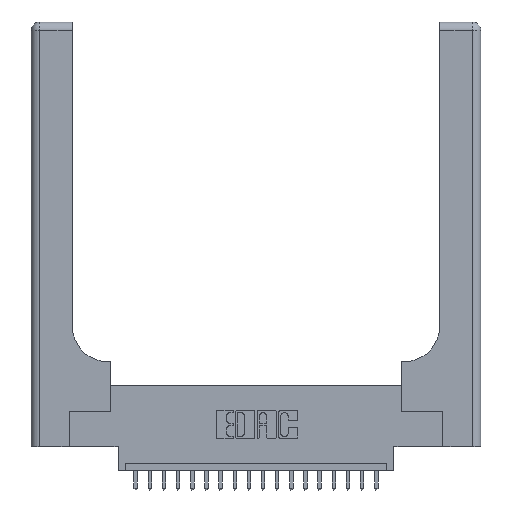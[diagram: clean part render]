
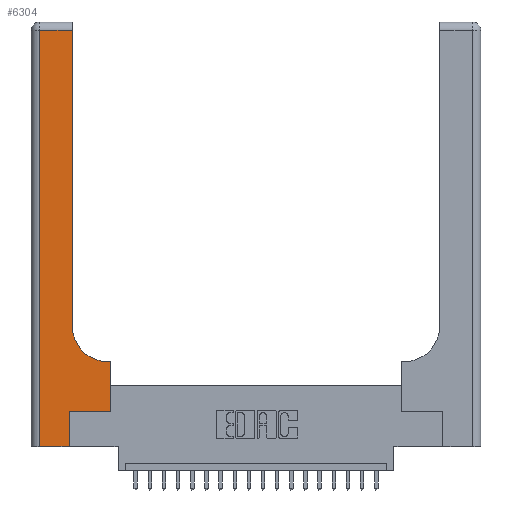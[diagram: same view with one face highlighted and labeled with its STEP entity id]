
A CAD part, top view. The second image highlights one B-rep face of the part: STEP entity #6304.
In plain terms, the highlighted planar face has unit normal (0, 0, 1).
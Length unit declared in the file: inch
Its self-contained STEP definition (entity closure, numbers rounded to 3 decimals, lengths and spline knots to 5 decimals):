
#1231 = CARTESIAN_POINT ( 'NONE',  ( 0.2915, 0.6, 0.37 ) ) ;
#1843 = CARTESIAN_POINT ( 'NONE',  ( 0.5585, 0.25, 0.37 ) ) ;
#1884 = DIRECTION ( 'NONE',  ( 1., 0., 0. ) ) ;
#3087 = VERTEX_POINT ( 'NONE', #7261 ) ;
#3095 = CARTESIAN_POINT ( 'NONE',  ( 0., 0., 0.37 ) ) ;
#3444 = EDGE_CURVE ( 'NONE', #20006, #18761, #9945, .T. ) ;
#3661 = ORIENTED_EDGE ( 'NONE', *, *, #21456, .T. ) ;
#4259 = EDGE_CURVE ( 'NONE', #7028, #18705, #18725, .T. ) ;
#4614 = VECTOR ( 'NONE', #9133, 39.37008 ) ;
#4795 = EDGE_CURVE ( 'NONE', #3087, #5387, #10986, .T. ) ;
#5135 = LINE ( 'NONE', #1843, #13689 ) ;
#5152 = EDGE_LOOP ( 'NONE', ( #8022, #11754, #18284, #7652, #18877, #15872, #3661, #17086, #14059 ) ) ;
#5387 = VERTEX_POINT ( 'NONE', #13367 ) ;
#5657 = VECTOR ( 'NONE', #9217, 39.37008 ) ;
#5728 = VERTEX_POINT ( 'NONE', #8145 ) ;
#5735 = CARTESIAN_POINT ( 'NONE',  ( 0.2915, 3., 0.37 ) ) ;
#5755 = EDGE_CURVE ( 'NONE', #18761, #3087, #11507, .T. ) ;
#5797 = DIRECTION ( 'NONE',  ( -1., 0., 0. ) ) ;
#5877 = VECTOR ( 'NONE', #9684, 39.37008 ) ;
#6205 = VECTOR ( 'NONE', #18537, 39.37008 ) ;
#6304 = ADVANCED_FACE ( 'NONE', ( #13922 ), #12515, .F. ) ;
#7028 = VERTEX_POINT ( 'NONE', #10907 ) ;
#7101 = DIRECTION ( 'NONE',  ( 0., 1., 0. ) ) ;
#7230 = DIRECTION ( 'NONE',  ( 1., 0., 0. ) ) ;
#7261 = CARTESIAN_POINT ( 'NONE',  ( 0.269, 0., 0.37 ) ) ;
#7466 = CARTESIAN_POINT ( 'NONE',  ( 0.5415, 0.85, 0.37 ) ) ;
#7652 = ORIENTED_EDGE ( 'NONE', *, *, #5755, .T. ) ;
#8022 = ORIENTED_EDGE ( 'NONE', *, *, #4259, .T. ) ;
#8145 = CARTESIAN_POINT ( 'NONE',  ( 0.5415, 0.6, 0.37 ) ) ;
#8517 = VERTEX_POINT ( 'NONE', #21505 ) ;
#9133 = DIRECTION ( 'NONE',  ( 0., 1., 0. ) ) ;
#9148 = DIRECTION ( 'NONE',  ( 0., 0., -1. ) ) ;
#9217 = DIRECTION ( 'NONE',  ( 0., 1., 0. ) ) ;
#9305 = VERTEX_POINT ( 'NONE', #10525 ) ;
#9640 = CARTESIAN_POINT ( 'NONE',  ( 0.06, 0., 0.37 ) ) ;
#9684 = DIRECTION ( 'NONE',  ( -1., 0., 0. ) ) ;
#9945 = LINE ( 'NONE', #13618, #6205 ) ;
#10200 = CIRCLE ( 'NONE', #17585, 0.25 ) ;
#10267 = DIRECTION ( 'NONE',  ( -1., 0., 0. ) ) ;
#10525 = CARTESIAN_POINT ( 'NONE',  ( 0.5585, 0.6, 0.37 ) ) ;
#10907 = CARTESIAN_POINT ( 'NONE',  ( 0.2915, 0.85, 0.37 ) ) ;
#10986 = LINE ( 'NONE', #17590, #4614 ) ;
#11022 = DIRECTION ( 'NONE',  ( 0., 0., -1. ) ) ;
#11041 = CARTESIAN_POINT ( 'NONE',  ( 0.06, 2.94, 0.37 ) ) ;
#11507 = LINE ( 'NONE', #3095, #16042 ) ;
#11711 = EDGE_CURVE ( 'NONE', #9305, #5728, #20611, .T. ) ;
#11749 = CARTESIAN_POINT ( 'NONE',  ( 0., 3., 0.37 ) ) ;
#11754 = ORIENTED_EDGE ( 'NONE', *, *, #12599, .T. ) ;
#12015 = EDGE_CURVE ( 'NONE', #5387, #8517, #20897, .T. ) ;
#12515 = PLANE ( 'NONE',  #17218 ) ;
#12599 = EDGE_CURVE ( 'NONE', #18705, #20006, #18176, .T. ) ;
#13367 = CARTESIAN_POINT ( 'NONE',  ( 0.269, 0.25, 0.37 ) ) ;
#13618 = CARTESIAN_POINT ( 'NONE',  ( 0.06, 3., 0.37 ) ) ;
#13689 = VECTOR ( 'NONE', #7101, 39.37008 ) ;
#13922 = FACE_OUTER_BOUND ( 'NONE', #5152, .T. ) ;
#14059 = ORIENTED_EDGE ( 'NONE', *, *, #20931, .T. ) ;
#15872 = ORIENTED_EDGE ( 'NONE', *, *, #12015, .T. ) ;
#16042 = VECTOR ( 'NONE', #21688, 39.37008 ) ;
#17086 = ORIENTED_EDGE ( 'NONE', *, *, #11711, .T. ) ;
#17218 = AXIS2_PLACEMENT_3D ( 'NONE', #11749, #11022, #5797 ) ;
#17585 = AXIS2_PLACEMENT_3D ( 'NONE', #7466, #9148, #7230 ) ;
#17590 = CARTESIAN_POINT ( 'NONE',  ( 0.269, 0., 0.37 ) ) ;
#18176 = LINE ( 'NONE', #18867, #19808 ) ;
#18284 = ORIENTED_EDGE ( 'NONE', *, *, #3444, .T. ) ;
#18487 = VECTOR ( 'NONE', #1884, 39.37008 ) ;
#18537 = DIRECTION ( 'NONE',  ( 0., -1., 0. ) ) ;
#18705 = VERTEX_POINT ( 'NONE', #19229 ) ;
#18725 = LINE ( 'NONE', #5735, #5657 ) ;
#18761 = VERTEX_POINT ( 'NONE', #9640 ) ;
#18867 = CARTESIAN_POINT ( 'NONE',  ( 0., 2.94, 0.37 ) ) ;
#18877 = ORIENTED_EDGE ( 'NONE', *, *, #4795, .T. ) ;
#18950 = CARTESIAN_POINT ( 'NONE',  ( 0.269, 0.25, 0.37 ) ) ;
#19229 = CARTESIAN_POINT ( 'NONE',  ( 0.2915, 2.94, 0.37 ) ) ;
#19808 = VECTOR ( 'NONE', #10267, 39.37008 ) ;
#20006 = VERTEX_POINT ( 'NONE', #11041 ) ;
#20611 = LINE ( 'NONE', #1231, #5877 ) ;
#20897 = LINE ( 'NONE', #18950, #18487 ) ;
#20931 = EDGE_CURVE ( 'NONE', #5728, #7028, #10200, .T. ) ;
#21456 = EDGE_CURVE ( 'NONE', #8517, #9305, #5135, .T. ) ;
#21505 = CARTESIAN_POINT ( 'NONE',  ( 0.5585, 0.25, 0.37 ) ) ;
#21688 = DIRECTION ( 'NONE',  ( 1., 0., 0. ) ) ;
